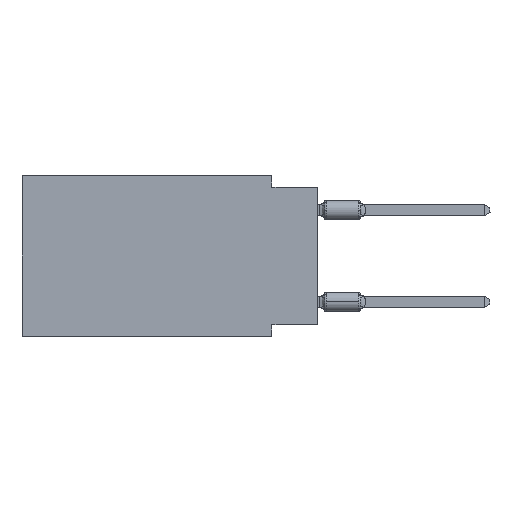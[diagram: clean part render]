
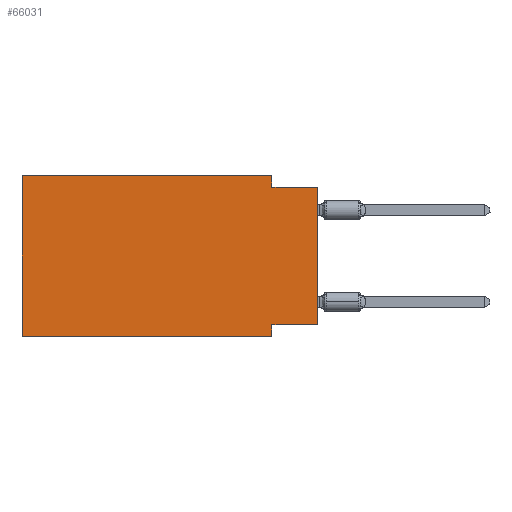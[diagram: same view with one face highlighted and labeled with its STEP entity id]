
A CAD part, left-side view. The second image highlights one B-rep face of the part: STEP entity #66031.
In plain terms, the highlighted planar face has unit normal (-1, 0, 0).
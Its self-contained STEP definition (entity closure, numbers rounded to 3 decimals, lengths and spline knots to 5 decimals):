
#973 = VERTEX_POINT ( 'NONE', #44491 ) ;
#1437 = EDGE_CURVE ( 'NONE', #49683, #24538, #66974, .T. ) ;
#1936 = LINE ( 'NONE', #69408, #15222 ) ;
#2382 = DIRECTION ( 'NONE',  ( 0., 0., -1. ) ) ;
#3291 = PLANE ( 'NONE',  #62158 ) ;
#4224 = CARTESIAN_POINT ( 'NONE',  ( 0., 0.645, -0.35 ) ) ;
#5823 = ORIENTED_EDGE ( 'NONE', *, *, #36574, .F. ) ;
#7533 = ORIENTED_EDGE ( 'NONE', *, *, #23924, .F. ) ;
#7764 = DIRECTION ( 'NONE',  ( 0., -1., 0. ) ) ;
#9097 = LINE ( 'NONE', #30259, #11945 ) ;
#9809 = VERTEX_POINT ( 'NONE', #31057 ) ;
#11945 = VECTOR ( 'NONE', #52515, 39.37008 ) ;
#13607 = DIRECTION ( 'NONE',  ( 0., 0., -1. ) ) ;
#15222 = VECTOR ( 'NONE', #13607, 39.37008 ) ;
#17029 = CARTESIAN_POINT ( 'NONE',  ( 0., 0.645, 0. ) ) ;
#17179 = CARTESIAN_POINT ( 'NONE',  ( 0., 0.1, -0.35 ) ) ;
#17844 = VERTEX_POINT ( 'NONE', #43856 ) ;
#18148 = ORIENTED_EDGE ( 'NONE', *, *, #1437, .F. ) ;
#19099 = CARTESIAN_POINT ( 'NONE',  ( 0., 0., -0.325 ) ) ;
#21638 = EDGE_CURVE ( 'NONE', #24538, #17844, #9097, .T. ) ;
#22511 = EDGE_LOOP ( 'NONE', ( #25940, #5823, #25455, #52501, #18148, #35266, #22869, #7533 ) ) ;
#22804 = DIRECTION ( 'NONE',  ( 0., 0., 1. ) ) ;
#22869 = ORIENTED_EDGE ( 'NONE', *, *, #41868, .F. ) ;
#23924 = EDGE_CURVE ( 'NONE', #27006, #9809, #33892, .T. ) ;
#24538 = VERTEX_POINT ( 'NONE', #71656 ) ;
#24593 = EDGE_CURVE ( 'NONE', #49683, #43723, #58947, .T. ) ;
#25455 = ORIENTED_EDGE ( 'NONE', *, *, #32126, .F. ) ;
#25940 = ORIENTED_EDGE ( 'NONE', *, *, #53343, .T. ) ;
#26084 = VECTOR ( 'NONE', #7764, 39.37008 ) ;
#26361 = VECTOR ( 'NONE', #2382, 39.37008 ) ;
#27006 = VERTEX_POINT ( 'NONE', #19099 ) ;
#27680 = VECTOR ( 'NONE', #70252, 39.37008 ) ;
#27808 = DIRECTION ( 'NONE',  ( 0., 0., -1. ) ) ;
#30259 = CARTESIAN_POINT ( 'NONE',  ( 0., 0.645, 0. ) ) ;
#31057 = CARTESIAN_POINT ( 'NONE',  ( 0., 0.1, -0.325 ) ) ;
#32126 = EDGE_CURVE ( 'NONE', #17844, #55585, #1936, .T. ) ;
#33892 = LINE ( 'NONE', #44837, #43941 ) ;
#35266 = ORIENTED_EDGE ( 'NONE', *, *, #24593, .T. ) ;
#36228 = CARTESIAN_POINT ( 'NONE',  ( 0., 0., -0.025 ) ) ;
#36574 = EDGE_CURVE ( 'NONE', #55585, #973, #47900, .T. ) ;
#39269 = DIRECTION ( 'NONE',  ( 0., 0., 1. ) ) ;
#41868 = EDGE_CURVE ( 'NONE', #9809, #43723, #44071, .T. ) ;
#43611 = CARTESIAN_POINT ( 'NONE',  ( 0., 0.1, -0.025 ) ) ;
#43723 = VERTEX_POINT ( 'NONE', #17179 ) ;
#43856 = CARTESIAN_POINT ( 'NONE',  ( 0., 0.1, 0. ) ) ;
#43941 = VECTOR ( 'NONE', #55766, 39.37008 ) ;
#44071 = LINE ( 'NONE', #66304, #26361 ) ;
#44491 = CARTESIAN_POINT ( 'NONE',  ( 0., 0., -0.025 ) ) ;
#44837 = CARTESIAN_POINT ( 'NONE',  ( 0., 0., -0.325 ) ) ;
#46042 = CARTESIAN_POINT ( 'NONE',  ( 0., 0.645, 0. ) ) ;
#47900 = LINE ( 'NONE', #36228, #26084 ) ;
#49557 = CARTESIAN_POINT ( 'NONE',  ( 0., 0.645, -0.35 ) ) ;
#49683 = VERTEX_POINT ( 'NONE', #49557 ) ;
#52501 = ORIENTED_EDGE ( 'NONE', *, *, #21638, .F. ) ;
#52515 = DIRECTION ( 'NONE',  ( 0., -1., 0. ) ) ;
#53261 = FACE_OUTER_BOUND ( 'NONE', #22511, .T. ) ;
#53343 = EDGE_CURVE ( 'NONE', #27006, #973, #55997, .T. ) ;
#55585 = VERTEX_POINT ( 'NONE', #43611 ) ;
#55766 = DIRECTION ( 'NONE',  ( 0., 1., 0. ) ) ;
#55997 = LINE ( 'NONE', #62909, #68658 ) ;
#58947 = LINE ( 'NONE', #4224, #27680 ) ;
#62158 = AXIS2_PLACEMENT_3D ( 'NONE', #46042, #68262, #27808 ) ;
#62909 = CARTESIAN_POINT ( 'NONE',  ( 0., 0., 0. ) ) ;
#66031 = ADVANCED_FACE ( 'NONE', ( #53261 ), #3291, .F. ) ;
#66304 = CARTESIAN_POINT ( 'NONE',  ( 0., 0.1, -0.35 ) ) ;
#66974 = LINE ( 'NONE', #17029, #70142 ) ;
#68262 = DIRECTION ( 'NONE',  ( 1., 0., 0. ) ) ;
#68658 = VECTOR ( 'NONE', #22804, 39.37008 ) ;
#69408 = CARTESIAN_POINT ( 'NONE',  ( 0., 0.1, 0. ) ) ;
#70142 = VECTOR ( 'NONE', #39269, 39.37008 ) ;
#70252 = DIRECTION ( 'NONE',  ( 0., -1., 0. ) ) ;
#71656 = CARTESIAN_POINT ( 'NONE',  ( 0., 0.645, 0. ) ) ;
